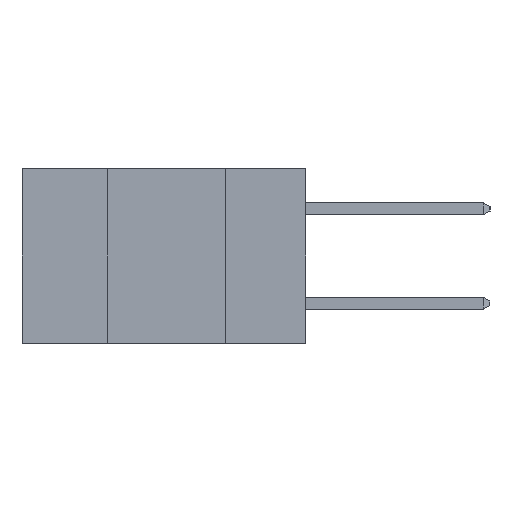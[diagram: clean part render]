
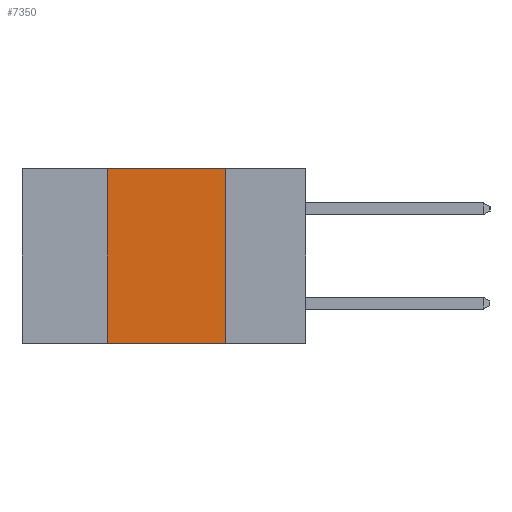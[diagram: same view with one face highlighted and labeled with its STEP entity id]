
A CAD part, left-side view. The second image highlights one B-rep face of the part: STEP entity #7350.
In plain terms, the highlighted planar face has unit normal (-1, 0, 0).
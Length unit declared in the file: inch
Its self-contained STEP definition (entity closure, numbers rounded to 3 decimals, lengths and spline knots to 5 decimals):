
#144 = VECTOR ( 'NONE', #4622, 39.37008 ) ;
#1034 = DIRECTION ( 'NONE',  ( 0., -1., 0. ) ) ;
#1108 = LINE ( 'NONE', #6827, #7994 ) ;
#1258 = VERTEX_POINT ( 'NONE', #8215 ) ;
#2659 = EDGE_CURVE ( 'NONE', #1258, #9580, #5272, .T. ) ;
#2948 = ORIENTED_EDGE ( 'NONE', *, *, #13135, .T. ) ;
#4622 = DIRECTION ( 'NONE',  ( 0., 0., -1. ) ) ;
#5272 = LINE ( 'NONE', #11110, #11201 ) ;
#5606 = CARTESIAN_POINT ( 'NONE',  ( 0., 0.17, -0.37 ) ) ;
#6322 = ORIENTED_EDGE ( 'NONE', *, *, #10325, .F. ) ;
#6452 = ORIENTED_EDGE ( 'NONE', *, *, #12852, .F. ) ;
#6459 = VECTOR ( 'NONE', #10907, 39.37008 ) ;
#6827 = CARTESIAN_POINT ( 'NONE',  ( 0., 0.6, 0. ) ) ;
#6922 = EDGE_LOOP ( 'NONE', ( #6452, #6322, #7942, #2948 ) ) ;
#7309 = FACE_OUTER_BOUND ( 'NONE', #6922, .T. ) ;
#7350 = ADVANCED_FACE ( 'NONE', ( #7309 ), #9655, .F. ) ;
#7462 = DIRECTION ( 'NONE',  ( 1., 0., 0. ) ) ;
#7891 = AXIS2_PLACEMENT_3D ( 'NONE', #8588, #7462, #13027 ) ;
#7942 = ORIENTED_EDGE ( 'NONE', *, *, #2659, .F. ) ;
#7994 = VECTOR ( 'NONE', #1034, 39.37008 ) ;
#8215 = CARTESIAN_POINT ( 'NONE',  ( 0., 0.42, -0.37 ) ) ;
#8588 = CARTESIAN_POINT ( 'NONE',  ( 0., 0.6, 0. ) ) ;
#9028 = LINE ( 'NONE', #5606, #144 ) ;
#9580 = VERTEX_POINT ( 'NONE', #11726 ) ;
#9655 = PLANE ( 'NONE',  #7891 ) ;
#9687 = LINE ( 'NONE', #9916, #6459 ) ;
#9916 = CARTESIAN_POINT ( 'NONE',  ( 0., 0.6, -0.37 ) ) ;
#10049 = DIRECTION ( 'NONE',  ( 0., 0., 1. ) ) ;
#10204 = VERTEX_POINT ( 'NONE', #14649 ) ;
#10325 = EDGE_CURVE ( 'NONE', #9580, #13980, #1108, .T. ) ;
#10907 = DIRECTION ( 'NONE',  ( 0., -1., 0. ) ) ;
#11110 = CARTESIAN_POINT ( 'NONE',  ( 0., 0.42, -0.37 ) ) ;
#11201 = VECTOR ( 'NONE', #10049, 39.37008 ) ;
#11726 = CARTESIAN_POINT ( 'NONE',  ( 0., 0.42, 0. ) ) ;
#12852 = EDGE_CURVE ( 'NONE', #13980, #10204, #9028, .T. ) ;
#12859 = CARTESIAN_POINT ( 'NONE',  ( 0., 0.17, 0. ) ) ;
#13027 = DIRECTION ( 'NONE',  ( 0., 0., -1. ) ) ;
#13135 = EDGE_CURVE ( 'NONE', #1258, #10204, #9687, .T. ) ;
#13980 = VERTEX_POINT ( 'NONE', #12859 ) ;
#14649 = CARTESIAN_POINT ( 'NONE',  ( 0., 0.17, -0.37 ) ) ;
